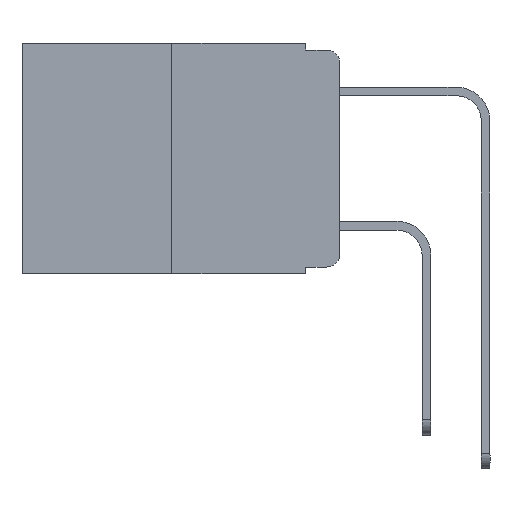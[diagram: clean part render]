
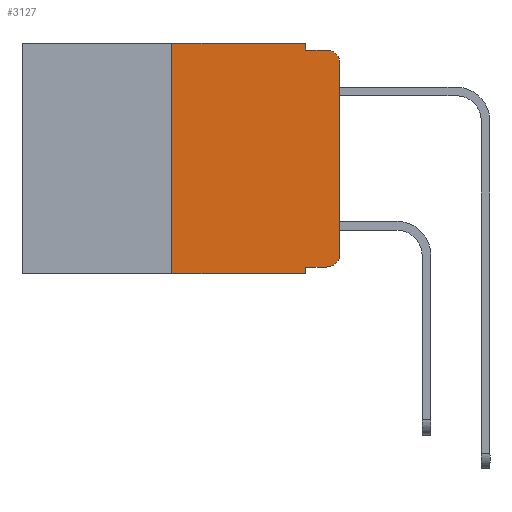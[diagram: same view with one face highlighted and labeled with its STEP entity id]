
A CAD part, left-side view. The second image highlights one B-rep face of the part: STEP entity #3127.
In plain terms, the highlighted planar face has unit normal (-1, 0, 0).
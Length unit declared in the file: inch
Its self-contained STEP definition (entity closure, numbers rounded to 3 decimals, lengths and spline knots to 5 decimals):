
#133 = EDGE_LOOP ( 'NONE', ( #10603, #782, #12327, #8402, #1758, #9930, #6205, #4296, #2764, #5406 ) ) ;
#140 = CIRCLE ( 'NONE', #3124, 0.02 ) ;
#258 = VECTOR ( 'NONE', #315, 39.37008 ) ;
#315 = DIRECTION ( 'NONE',  ( 0., 0., -1. ) ) ;
#527 = EDGE_CURVE ( 'NONE', #8541, #10417, #1652, .T. ) ;
#544 = CARTESIAN_POINT ( 'NONE',  ( 0., 0.25, 0. ) ) ;
#782 = ORIENTED_EDGE ( 'NONE', *, *, #527, .T. ) ;
#973 = CARTESIAN_POINT ( 'NONE',  ( 0., 0.02, -0.03 ) ) ;
#1181 = CARTESIAN_POINT ( 'NONE',  ( 0., 0.051, -0.343 ) ) ;
#1623 = EDGE_CURVE ( 'NONE', #7393, #5762, #11124, .T. ) ;
#1652 = CIRCLE ( 'NONE', #2460, 0.02 ) ;
#1694 = VECTOR ( 'NONE', #2474, 39.37008 ) ;
#1758 = ORIENTED_EDGE ( 'NONE', *, *, #7828, .F. ) ;
#1925 = CARTESIAN_POINT ( 'NONE',  ( 0., 0.25, 0. ) ) ;
#1976 = DIRECTION ( 'NONE',  ( 0., 0., -1. ) ) ;
#2061 = EDGE_CURVE ( 'NONE', #11230, #5950, #8148, .T. ) ;
#2170 = DIRECTION ( 'NONE',  ( 0., 0., 1. ) ) ;
#2291 = CARTESIAN_POINT ( 'NONE',  ( 0., 0.051, 0. ) ) ;
#2460 = AXIS2_PLACEMENT_3D ( 'NONE', #973, #8717, #1976 ) ;
#2474 = DIRECTION ( 'NONE',  ( 0., -1., 0. ) ) ;
#2635 = CARTESIAN_POINT ( 'NONE',  ( 0., 0.051, -0.01 ) ) ;
#2764 = ORIENTED_EDGE ( 'NONE', *, *, #4312, .T. ) ;
#2802 = DIRECTION ( 'NONE',  ( 0., -1., 0. ) ) ;
#2869 = CARTESIAN_POINT ( 'NONE',  ( 0., 0.02, -0.01 ) ) ;
#3124 = AXIS2_PLACEMENT_3D ( 'NONE', #7504, #10590, #11531 ) ;
#3127 = ADVANCED_FACE ( 'NONE', ( #6657 ), #5718, .F. ) ;
#3534 = AXIS2_PLACEMENT_3D ( 'NONE', #8400, #7400, #10228 ) ;
#3574 = CARTESIAN_POINT ( 'NONE',  ( 0., 0.02, -0.333 ) ) ;
#3761 = EDGE_CURVE ( 'NONE', #8533, #6853, #140, .T. ) ;
#4095 = CARTESIAN_POINT ( 'NONE',  ( 0., 0.051, -0.333 ) ) ;
#4296 = ORIENTED_EDGE ( 'NONE', *, *, #1623, .F. ) ;
#4312 = EDGE_CURVE ( 'NONE', #7393, #8533, #6857, .T. ) ;
#4419 = VECTOR ( 'NONE', #2802, 39.37008 ) ;
#4833 = VECTOR ( 'NONE', #2170, 39.37008 ) ;
#5019 = VECTOR ( 'NONE', #9479, 39.37008 ) ;
#5406 = ORIENTED_EDGE ( 'NONE', *, *, #3761, .T. ) ;
#5718 = PLANE ( 'NONE',  #3534 ) ;
#5762 = VERTEX_POINT ( 'NONE', #1181 ) ;
#5950 = VERTEX_POINT ( 'NONE', #2635 ) ;
#6200 = DIRECTION ( 'NONE',  ( 0., 0., -1. ) ) ;
#6205 = ORIENTED_EDGE ( 'NONE', *, *, #10527, .T. ) ;
#6389 = EDGE_CURVE ( 'NONE', #5950, #10417, #11315, .T. ) ;
#6657 = FACE_OUTER_BOUND ( 'NONE', #133, .T. ) ;
#6759 = CARTESIAN_POINT ( 'NONE',  ( 0., 0.25, -0.343 ) ) ;
#6853 = VERTEX_POINT ( 'NONE', #8495 ) ;
#6857 = LINE ( 'NONE', #4095, #8007 ) ;
#7029 = LINE ( 'NONE', #544, #8323 ) ;
#7233 = EDGE_CURVE ( 'NONE', #6853, #8541, #11686, .T. ) ;
#7393 = VERTEX_POINT ( 'NONE', #11562 ) ;
#7400 = DIRECTION ( 'NONE',  ( 1., 0., 0. ) ) ;
#7504 = CARTESIAN_POINT ( 'NONE',  ( 0., 0.02, -0.313 ) ) ;
#7769 = CARTESIAN_POINT ( 'NONE',  ( 0., 0.473, 0. ) ) ;
#7828 = EDGE_CURVE ( 'NONE', #10365, #11230, #9599, .T. ) ;
#7910 = CARTESIAN_POINT ( 'NONE',  ( 0., 0., 0. ) ) ;
#7966 = LINE ( 'NONE', #9980, #1694 ) ;
#8007 = VECTOR ( 'NONE', #9818, 39.37008 ) ;
#8061 = VECTOR ( 'NONE', #6200, 39.37008 ) ;
#8148 = LINE ( 'NONE', #2291, #8061 ) ;
#8323 = VECTOR ( 'NONE', #9988, 39.37008 ) ;
#8400 = CARTESIAN_POINT ( 'NONE',  ( 0., 0.473, 0. ) ) ;
#8402 = ORIENTED_EDGE ( 'NONE', *, *, #2061, .F. ) ;
#8495 = CARTESIAN_POINT ( 'NONE',  ( 0., 0., -0.313 ) ) ;
#8533 = VERTEX_POINT ( 'NONE', #3574 ) ;
#8541 = VERTEX_POINT ( 'NONE', #9428 ) ;
#8717 = DIRECTION ( 'NONE',  ( -1., 0., 0. ) ) ;
#8778 = EDGE_CURVE ( 'NONE', #12229, #10365, #7029, .T. ) ;
#9167 = CARTESIAN_POINT ( 'NONE',  ( 0., 0.051, 0. ) ) ;
#9417 = CARTESIAN_POINT ( 'NONE',  ( 0., 0.051, -0.01 ) ) ;
#9428 = CARTESIAN_POINT ( 'NONE',  ( 0., 0., -0.03 ) ) ;
#9479 = DIRECTION ( 'NONE',  ( 0., -1., 0. ) ) ;
#9599 = LINE ( 'NONE', #7769, #5019 ) ;
#9818 = DIRECTION ( 'NONE',  ( 0., -1., 0. ) ) ;
#9930 = ORIENTED_EDGE ( 'NONE', *, *, #8778, .F. ) ;
#9980 = CARTESIAN_POINT ( 'NONE',  ( 0., 0.473, -0.343 ) ) ;
#9988 = DIRECTION ( 'NONE',  ( 0., 0., 1. ) ) ;
#10228 = DIRECTION ( 'NONE',  ( 0., 0., -1. ) ) ;
#10365 = VERTEX_POINT ( 'NONE', #1925 ) ;
#10417 = VERTEX_POINT ( 'NONE', #2869 ) ;
#10527 = EDGE_CURVE ( 'NONE', #12229, #5762, #7966, .T. ) ;
#10590 = DIRECTION ( 'NONE',  ( -1., 0., 0. ) ) ;
#10603 = ORIENTED_EDGE ( 'NONE', *, *, #7233, .T. ) ;
#11124 = LINE ( 'NONE', #9167, #258 ) ;
#11230 = VERTEX_POINT ( 'NONE', #12339 ) ;
#11315 = LINE ( 'NONE', #9417, #4419 ) ;
#11531 = DIRECTION ( 'NONE',  ( 0., 0., -1. ) ) ;
#11562 = CARTESIAN_POINT ( 'NONE',  ( 0., 0.051, -0.333 ) ) ;
#11686 = LINE ( 'NONE', #7910, #4833 ) ;
#12229 = VERTEX_POINT ( 'NONE', #6759 ) ;
#12327 = ORIENTED_EDGE ( 'NONE', *, *, #6389, .F. ) ;
#12339 = CARTESIAN_POINT ( 'NONE',  ( 0., 0.051, 0. ) ) ;
